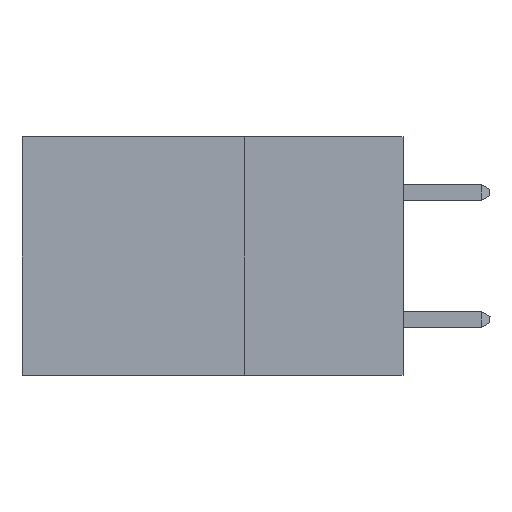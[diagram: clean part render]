
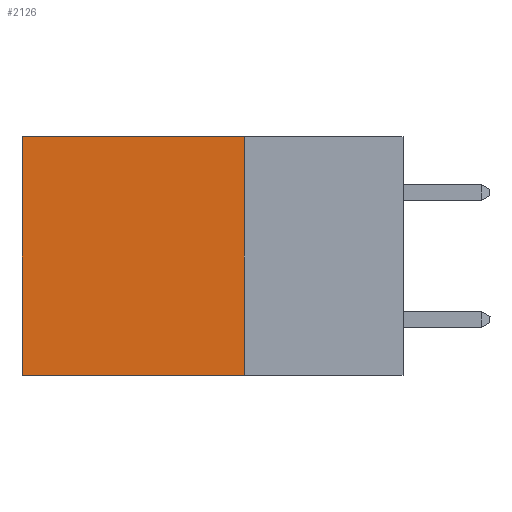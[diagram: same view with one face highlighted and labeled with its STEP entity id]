
A CAD part, left-side view. The second image highlights one B-rep face of the part: STEP entity #2126.
In plain terms, the highlighted planar face has unit normal (-1, 0, 0).
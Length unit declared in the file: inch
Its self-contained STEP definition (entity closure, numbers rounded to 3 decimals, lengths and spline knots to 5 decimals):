
#248 = DIRECTION ( 'NONE',  ( 0., 1., 0. ) ) ;
#679 = VERTEX_POINT ( 'NONE', #10113 ) ;
#692 = VECTOR ( 'NONE', #7824, 39.37008 ) ;
#720 = ORIENTED_EDGE ( 'NONE', *, *, #14966, .T. ) ;
#851 = VECTOR ( 'NONE', #248, 39.37008 ) ;
#1993 = CARTESIAN_POINT ( 'NONE',  ( 0.2875, 0.25, -0.375 ) ) ;
#2126 = ADVANCED_FACE ( 'NONE', ( #14553 ), #11836, .F. ) ;
#2417 = CARTESIAN_POINT ( 'NONE',  ( 0.2875, 0.6, 0. ) ) ;
#2795 = CARTESIAN_POINT ( 'NONE',  ( 0.2875, 0.25, -0.375 ) ) ;
#2891 = EDGE_LOOP ( 'NONE', ( #13855, #3460, #4125, #720 ) ) ;
#2908 = VERTEX_POINT ( 'NONE', #2417 ) ;
#3460 = ORIENTED_EDGE ( 'NONE', *, *, #3570, .F. ) ;
#3570 = EDGE_CURVE ( 'NONE', #13235, #679, #6502, .T. ) ;
#3691 = VECTOR ( 'NONE', #11618, 39.37008 ) ;
#4125 = ORIENTED_EDGE ( 'NONE', *, *, #12662, .F. ) ;
#4608 = DIRECTION ( 'NONE',  ( 1., 0., 0. ) ) ;
#5006 = LINE ( 'NONE', #1993, #3691 ) ;
#6120 = VECTOR ( 'NONE', #11306, 39.37008 ) ;
#6135 = CARTESIAN_POINT ( 'NONE',  ( 0.2875, 0.25, 0. ) ) ;
#6502 = LINE ( 'NONE', #2795, #6120 ) ;
#6586 = CARTESIAN_POINT ( 'NONE',  ( 0.2875, 0.6, -0.375 ) ) ;
#7094 = CARTESIAN_POINT ( 'NONE',  ( 0.2875, 0.25, -0.375 ) ) ;
#7824 = DIRECTION ( 'NONE',  ( 0., 0., -1. ) ) ;
#8118 = LINE ( 'NONE', #6586, #692 ) ;
#9810 = EDGE_CURVE ( 'NONE', #2908, #679, #8118, .T. ) ;
#10113 = CARTESIAN_POINT ( 'NONE',  ( 0.2875, 0.6, -0.375 ) ) ;
#11306 = DIRECTION ( 'NONE',  ( 0., 1., 0. ) ) ;
#11618 = DIRECTION ( 'NONE',  ( 0., 0., -1. ) ) ;
#11836 = PLANE ( 'NONE',  #14621 ) ;
#12594 = CARTESIAN_POINT ( 'NONE',  ( 0.2875, 0.25, -0.375 ) ) ;
#12628 = LINE ( 'NONE', #13533, #851 ) ;
#12662 = EDGE_CURVE ( 'NONE', #14381, #13235, #5006, .T. ) ;
#13235 = VERTEX_POINT ( 'NONE', #12594 ) ;
#13533 = CARTESIAN_POINT ( 'NONE',  ( 0.2875, 0.25, 0. ) ) ;
#13855 = ORIENTED_EDGE ( 'NONE', *, *, #9810, .T. ) ;
#14381 = VERTEX_POINT ( 'NONE', #6135 ) ;
#14387 = DIRECTION ( 'NONE',  ( 0., 0., -1. ) ) ;
#14553 = FACE_OUTER_BOUND ( 'NONE', #2891, .T. ) ;
#14621 = AXIS2_PLACEMENT_3D ( 'NONE', #7094, #4608, #14387 ) ;
#14966 = EDGE_CURVE ( 'NONE', #14381, #2908, #12628, .T. ) ;
